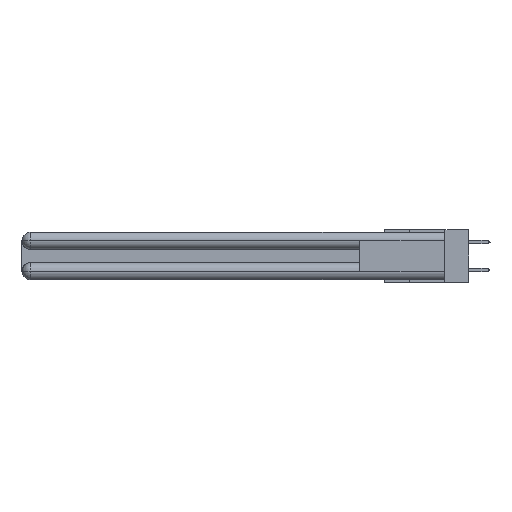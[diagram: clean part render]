
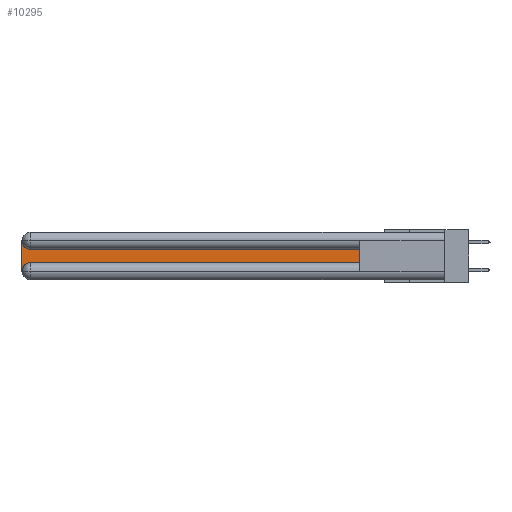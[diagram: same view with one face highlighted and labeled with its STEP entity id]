
A CAD part, left-side view. The second image highlights one B-rep face of the part: STEP entity #10295.
In plain terms, the highlighted planar face has unit normal (-1, 0, 0).
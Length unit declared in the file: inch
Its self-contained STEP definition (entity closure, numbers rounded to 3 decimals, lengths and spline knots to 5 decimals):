
#79 = PLANE ( 'NONE',  #21631 ) ;
#324 = CIRCLE ( 'NONE', #7381, 0.06 ) ;
#797 = LINE ( 'NONE', #17676, #17494 ) ;
#977 = CARTESIAN_POINT ( 'NONE',  ( 0.075, 2.94, -0.2775 ) ) ;
#2219 = CARTESIAN_POINT ( 'NONE',  ( 0.075, 0.6, -0.1225 ) ) ;
#2997 = FACE_OUTER_BOUND ( 'NONE', #22703, .T. ) ;
#3081 = CARTESIAN_POINT ( 'NONE',  ( 0.075, 2.94, -0.2175 ) ) ;
#4008 = ORIENTED_EDGE ( 'NONE', *, *, #10401, .T. ) ;
#4420 = LINE ( 'NONE', #16974, #5393 ) ;
#4685 = LINE ( 'NONE', #25894, #26375 ) ;
#5175 = EDGE_CURVE ( 'NONE', #11150, #17101, #4420, .T. ) ;
#5393 = VECTOR ( 'NONE', #27496, 39.37008 ) ;
#5792 = ORIENTED_EDGE ( 'NONE', *, *, #9564, .T. ) ;
#7381 = AXIS2_PLACEMENT_3D ( 'NONE', #19478, #17083, #24220 ) ;
#8744 = VECTOR ( 'NONE', #14825, 39.37008 ) ;
#9466 = ORIENTED_EDGE ( 'NONE', *, *, #16333, .T. ) ;
#9564 = EDGE_CURVE ( 'NONE', #14462, #23748, #19108, .T. ) ;
#10295 = ADVANCED_FACE ( 'NONE', ( #2997 ), #79, .F. ) ;
#10401 = EDGE_CURVE ( 'NONE', #17101, #14462, #4685, .T. ) ;
#11150 = VERTEX_POINT ( 'NONE', #3081 ) ;
#12647 = CARTESIAN_POINT ( 'NONE',  ( 0.075, 2.94, -0.1225 ) ) ;
#13269 = AXIS2_PLACEMENT_3D ( 'NONE', #977, #15900, #16185 ) ;
#14462 = VERTEX_POINT ( 'NONE', #2219 ) ;
#14825 = DIRECTION ( 'NONE',  ( 0., 1., 0. ) ) ;
#15171 = VERTEX_POINT ( 'NONE', #22187 ) ;
#15900 = DIRECTION ( 'NONE',  ( 1., 0., 0. ) ) ;
#16185 = DIRECTION ( 'NONE',  ( 0., 0., -1. ) ) ;
#16333 = EDGE_CURVE ( 'NONE', #16794, #15171, #797, .T. ) ;
#16794 = VERTEX_POINT ( 'NONE', #24974 ) ;
#16974 = CARTESIAN_POINT ( 'NONE',  ( 0.075, 0.6, -0.2175 ) ) ;
#17004 = CARTESIAN_POINT ( 'NONE',  ( 0.075, 0.6, -0.1225 ) ) ;
#17083 = DIRECTION ( 'NONE',  ( 1., 0., 0. ) ) ;
#17101 = VERTEX_POINT ( 'NONE', #18147 ) ;
#17163 = DIRECTION ( 'NONE',  ( 1., 0., 0. ) ) ;
#17494 = VECTOR ( 'NONE', #18694, 39.37008 ) ;
#17676 = CARTESIAN_POINT ( 'NONE',  ( 0.075, 3., -0.2175 ) ) ;
#18147 = CARTESIAN_POINT ( 'NONE',  ( 0.075, 0.6, -0.2175 ) ) ;
#18694 = DIRECTION ( 'NONE',  ( 0., 0., -1. ) ) ;
#18932 = CARTESIAN_POINT ( 'NONE',  ( 0.075, 3., -0.1225 ) ) ;
#19108 = LINE ( 'NONE', #17004, #8744 ) ;
#19478 = CARTESIAN_POINT ( 'NONE',  ( 0.075, 2.94, -0.0625 ) ) ;
#20031 = ORIENTED_EDGE ( 'NONE', *, *, #22068, .T. ) ;
#21631 = AXIS2_PLACEMENT_3D ( 'NONE', #18932, #17163, #27409 ) ;
#22068 = EDGE_CURVE ( 'NONE', #15171, #11150, #23702, .T. ) ;
#22187 = CARTESIAN_POINT ( 'NONE',  ( 0.075, 3., -0.2775 ) ) ;
#22592 = ORIENTED_EDGE ( 'NONE', *, *, #5175, .T. ) ;
#22703 = EDGE_LOOP ( 'NONE', ( #5792, #23225, #9466, #20031, #22592, #4008 ) ) ;
#23225 = ORIENTED_EDGE ( 'NONE', *, *, #23892, .T. ) ;
#23702 = CIRCLE ( 'NONE', #13269, 0.06 ) ;
#23748 = VERTEX_POINT ( 'NONE', #12647 ) ;
#23892 = EDGE_CURVE ( 'NONE', #23748, #16794, #324, .T. ) ;
#23956 = DIRECTION ( 'NONE',  ( 0., 0., 1. ) ) ;
#24220 = DIRECTION ( 'NONE',  ( 0., 0., -1. ) ) ;
#24974 = CARTESIAN_POINT ( 'NONE',  ( 0.075, 3., -0.0625 ) ) ;
#25894 = CARTESIAN_POINT ( 'NONE',  ( 0.075, 0.6, -0.2175 ) ) ;
#26375 = VECTOR ( 'NONE', #23956, 39.37008 ) ;
#27409 = DIRECTION ( 'NONE',  ( 0., 0., -1. ) ) ;
#27496 = DIRECTION ( 'NONE',  ( 0., -1., 0. ) ) ;
